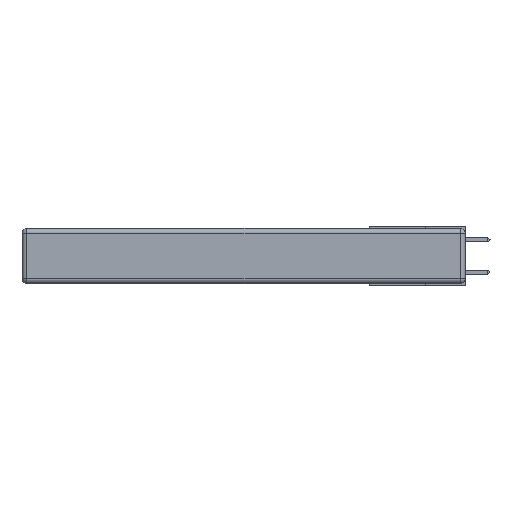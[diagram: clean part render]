
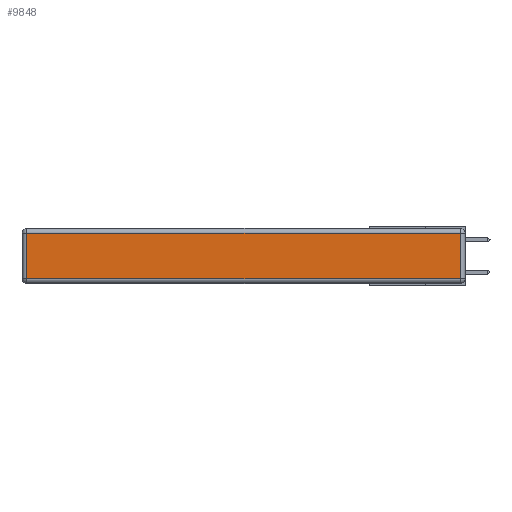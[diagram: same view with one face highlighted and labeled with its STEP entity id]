
A CAD part, left-side view. The second image highlights one B-rep face of the part: STEP entity #9848.
In plain terms, the highlighted planar face has unit normal (-1, 0, 0).
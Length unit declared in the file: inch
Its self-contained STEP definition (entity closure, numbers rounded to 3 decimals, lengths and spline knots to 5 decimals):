
#46 = LINE ( 'NONE', #6046, #1070 ) ;
#97 = DIRECTION ( 'NONE',  ( -1., 0., 0. ) ) ;
#1029 = DIRECTION ( 'NONE',  ( 0., -1., 0. ) ) ;
#1070 = VECTOR ( 'NONE', #1752, 39.37008 ) ;
#1090 = PLANE ( 'NONE',  #7184 ) ;
#1182 = CARTESIAN_POINT ( 'NONE',  ( 0., 0., -0.343 ) ) ;
#1752 = DIRECTION ( 'NONE',  ( 0., 1., 0. ) ) ;
#1973 = VERTEX_POINT ( 'NONE', #7203 ) ;
#3659 = VERTEX_POINT ( 'NONE', #4002 ) ;
#3737 = ORIENTED_EDGE ( 'NONE', *, *, #7164, .T. ) ;
#4002 = CARTESIAN_POINT ( 'NONE',  ( 0., 2.72, -0.313 ) ) ;
#4054 = ORIENTED_EDGE ( 'NONE', *, *, #13092, .T. ) ;
#4190 = LINE ( 'NONE', #5084, #6597 ) ;
#5084 = CARTESIAN_POINT ( 'NONE',  ( 0., 2.72, -0.343 ) ) ;
#5893 = LINE ( 'NONE', #13539, #11336 ) ;
#6046 = CARTESIAN_POINT ( 'NONE',  ( 0., 2.75, -0.03 ) ) ;
#6361 = FACE_OUTER_BOUND ( 'NONE', #12007, .T. ) ;
#6416 = EDGE_CURVE ( 'NONE', #3659, #13830, #13559, .T. ) ;
#6597 = VECTOR ( 'NONE', #10653, 39.37008 ) ;
#7164 = EDGE_CURVE ( 'NONE', #1973, #3659, #4190, .T. ) ;
#7184 = AXIS2_PLACEMENT_3D ( 'NONE', #1182, #97, #12015 ) ;
#7203 = CARTESIAN_POINT ( 'NONE',  ( 0., 2.72, -0.03 ) ) ;
#7281 = CARTESIAN_POINT ( 'NONE',  ( 0., 0.03, -0.313 ) ) ;
#9848 = ADVANCED_FACE ( 'NONE', ( #6361 ), #1090, .T. ) ;
#10344 = VERTEX_POINT ( 'NONE', #13921 ) ;
#10386 = DIRECTION ( 'NONE',  ( 0., 0., 1. ) ) ;
#10653 = DIRECTION ( 'NONE',  ( 0., 0., -1. ) ) ;
#11088 = ORIENTED_EDGE ( 'NONE', *, *, #6416, .T. ) ;
#11336 = VECTOR ( 'NONE', #10386, 39.37008 ) ;
#11354 = EDGE_CURVE ( 'NONE', #13830, #10344, #5893, .T. ) ;
#11400 = ORIENTED_EDGE ( 'NONE', *, *, #11354, .T. ) ;
#12007 = EDGE_LOOP ( 'NONE', ( #11088, #11400, #4054, #3737 ) ) ;
#12015 = DIRECTION ( 'NONE',  ( 0., 0., 1. ) ) ;
#12557 = VECTOR ( 'NONE', #1029, 39.37008 ) ;
#13092 = EDGE_CURVE ( 'NONE', #10344, #1973, #46, .T. ) ;
#13539 = CARTESIAN_POINT ( 'NONE',  ( 0., 0.03, -0.343 ) ) ;
#13559 = LINE ( 'NONE', #14017, #12557 ) ;
#13830 = VERTEX_POINT ( 'NONE', #7281 ) ;
#13921 = CARTESIAN_POINT ( 'NONE',  ( 0., 0.03, -0.03 ) ) ;
#14017 = CARTESIAN_POINT ( 'NONE',  ( 0., 0., -0.313 ) ) ;
